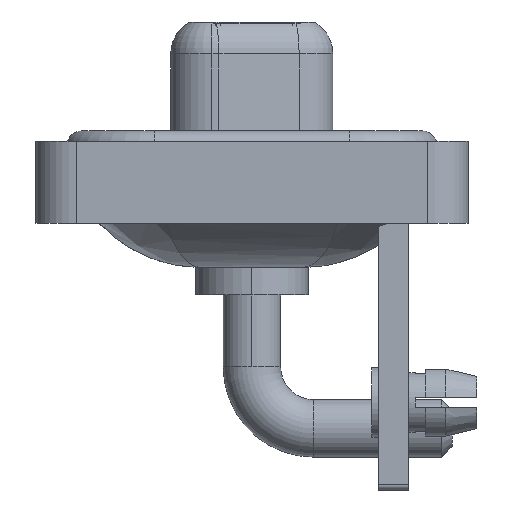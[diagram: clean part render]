
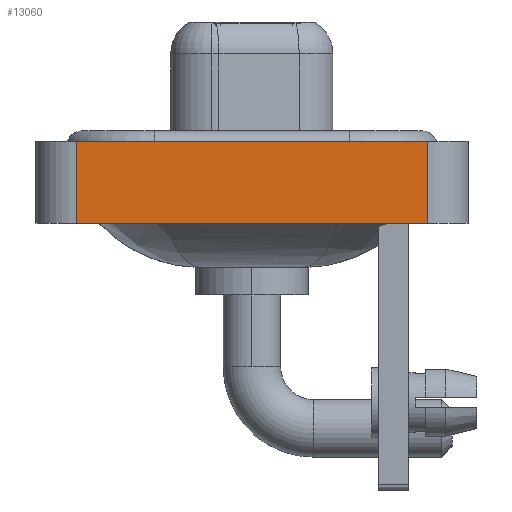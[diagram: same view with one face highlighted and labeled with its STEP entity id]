
A CAD part, left-side view. The second image highlights one B-rep face of the part: STEP entity #13060.
In plain terms, the highlighted planar face has unit normal (-1, 0, 0).
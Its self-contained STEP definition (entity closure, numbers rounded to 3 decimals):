
#833 = CARTESIAN_POINT ( 'NONE',  ( -7.25, -8.55, 0.4 ) ) ;
#969 = LINE ( 'NONE', #14893, #7427 ) ;
#2492 = DIRECTION ( 'NONE',  ( 0., 0., 1. ) ) ;
#3102 = DIRECTION ( 'NONE',  ( 0., 0., 1. ) ) ;
#3633 = VECTOR ( 'NONE', #11026, 1000. ) ;
#3867 = AXIS2_PLACEMENT_3D ( 'NONE', #16506, #15136, #2492 ) ;
#4194 = CARTESIAN_POINT ( 'NONE',  ( -7.25, -8.55, -3.6 ) ) ;
#4367 = LINE ( 'NONE', #4194, #10675 ) ;
#4560 = CARTESIAN_POINT ( 'NONE',  ( -7.25, 8.55, 0.4 ) ) ;
#5107 = DIRECTION ( 'NONE',  ( 0., -1., 0. ) ) ;
#5974 = VECTOR ( 'NONE', #3102, 1000. ) ;
#6306 = EDGE_LOOP ( 'NONE', ( #14576, #8192, #11162, #15173 ) ) ;
#7427 = VECTOR ( 'NONE', #5107, 1000. ) ;
#7653 = VERTEX_POINT ( 'NONE', #4560 ) ;
#8192 = ORIENTED_EDGE ( 'NONE', *, *, #16679, .F. ) ;
#10675 = VECTOR ( 'NONE', #15630, 1000. ) ;
#10847 = VERTEX_POINT ( 'NONE', #11815 ) ;
#10878 = PLANE ( 'NONE',  #3867 ) ;
#11026 = DIRECTION ( 'NONE',  ( 0., -1., 0. ) ) ;
#11029 = CARTESIAN_POINT ( 'NONE',  ( -7.25, -8.55, 0.4 ) ) ;
#11162 = ORIENTED_EDGE ( 'NONE', *, *, #16455, .F. ) ;
#11522 = VERTEX_POINT ( 'NONE', #11029 ) ;
#11815 = CARTESIAN_POINT ( 'NONE',  ( -7.25, 8.55, -3.6 ) ) ;
#12287 = LINE ( 'NONE', #17118, #5974 ) ;
#13060 = ADVANCED_FACE ( 'NONE', ( #13389 ), #10878, .T. ) ;
#13389 = FACE_OUTER_BOUND ( 'NONE', #6306, .T. ) ;
#13861 = EDGE_CURVE ( 'NONE', #10847, #16546, #969, .T. ) ;
#14576 = ORIENTED_EDGE ( 'NONE', *, *, #15723, .T. ) ;
#14893 = CARTESIAN_POINT ( 'NONE',  ( -7.25, -8.55, -3.6 ) ) ;
#15136 = DIRECTION ( 'NONE',  ( -1., 0., 0. ) ) ;
#15173 = ORIENTED_EDGE ( 'NONE', *, *, #13861, .T. ) ;
#15391 = CARTESIAN_POINT ( 'NONE',  ( -7.25, -8.55, -3.6 ) ) ;
#15630 = DIRECTION ( 'NONE',  ( 0., 0., 1. ) ) ;
#15723 = EDGE_CURVE ( 'NONE', #16546, #11522, #4367, .T. ) ;
#16455 = EDGE_CURVE ( 'NONE', #10847, #7653, #12287, .T. ) ;
#16485 = LINE ( 'NONE', #833, #3633 ) ;
#16506 = CARTESIAN_POINT ( 'NONE',  ( -7.25, -8.55, -3.6 ) ) ;
#16546 = VERTEX_POINT ( 'NONE', #15391 ) ;
#16679 = EDGE_CURVE ( 'NONE', #7653, #11522, #16485, .T. ) ;
#17118 = CARTESIAN_POINT ( 'NONE',  ( -7.25, 8.55, -3.6 ) ) ;
